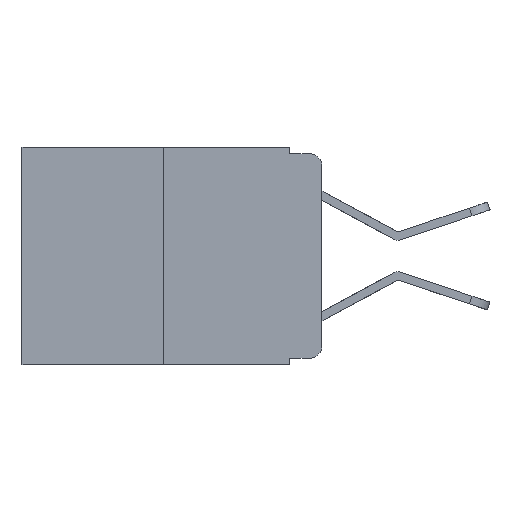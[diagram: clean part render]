
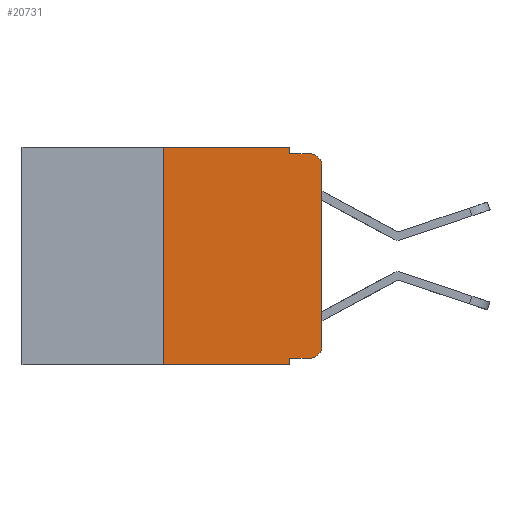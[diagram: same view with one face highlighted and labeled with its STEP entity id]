
A CAD part, left-side view. The second image highlights one B-rep face of the part: STEP entity #20731.
In plain terms, the highlighted planar face has unit normal (-1, 0, 0).
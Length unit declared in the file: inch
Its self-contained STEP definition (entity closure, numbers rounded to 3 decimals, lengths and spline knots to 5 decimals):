
#148 = VERTEX_POINT ( 'NONE', #4072 ) ;
#224 = DIRECTION ( 'NONE',  ( 0., 0., -1. ) ) ;
#341 = DIRECTION ( 'NONE',  ( 0., 0., -1. ) ) ;
#916 = VECTOR ( 'NONE', #18086, 39.37008 ) ;
#939 = EDGE_LOOP ( 'NONE', ( #4129, #20770, #5629, #3543, #6259, #16792, #4773, #17685, #23630, #23408 ) ) ;
#2148 = VERTEX_POINT ( 'NONE', #23301 ) ;
#2504 = LINE ( 'NONE', #6174, #8136 ) ;
#2553 = LINE ( 'NONE', #23036, #12594 ) ;
#3017 = CARTESIAN_POINT ( 'NONE',  ( 0., 0.473, 0. ) ) ;
#3543 = ORIENTED_EDGE ( 'NONE', *, *, #16401, .F. ) ;
#4072 = CARTESIAN_POINT ( 'NONE',  ( 0., 0.051, -0.01 ) ) ;
#4129 = ORIENTED_EDGE ( 'NONE', *, *, #15469, .T. ) ;
#4682 = VERTEX_POINT ( 'NONE', #21403 ) ;
#4773 = ORIENTED_EDGE ( 'NONE', *, *, #18448, .T. ) ;
#4928 = VERTEX_POINT ( 'NONE', #19489 ) ;
#4990 = AXIS2_PLACEMENT_3D ( 'NONE', #18432, #7250, #20255 ) ;
#5586 = VERTEX_POINT ( 'NONE', #23264 ) ;
#5629 = ORIENTED_EDGE ( 'NONE', *, *, #20079, .F. ) ;
#6174 = CARTESIAN_POINT ( 'NONE',  ( 0., 0.473, 0. ) ) ;
#6259 = ORIENTED_EDGE ( 'NONE', *, *, #19309, .F. ) ;
#6754 = VERTEX_POINT ( 'NONE', #23220 ) ;
#7192 = CIRCLE ( 'NONE', #4990, 0.02 ) ;
#7250 = DIRECTION ( 'NONE',  ( -1., 0., 0. ) ) ;
#8136 = VECTOR ( 'NONE', #15414, 39.37008 ) ;
#8357 = CARTESIAN_POINT ( 'NONE',  ( 0., 0.25, -0.343 ) ) ;
#8527 = EDGE_CURVE ( 'NONE', #14965, #6754, #18159, .T. ) ;
#8721 = DIRECTION ( 'NONE',  ( 0., 0., -1. ) ) ;
#9644 = CARTESIAN_POINT ( 'NONE',  ( 0., 0.051, 0. ) ) ;
#10605 = EDGE_CURVE ( 'NONE', #5586, #11191, #13725, .T. ) ;
#10972 = LINE ( 'NONE', #21681, #916 ) ;
#11020 = VECTOR ( 'NONE', #224, 39.37008 ) ;
#11191 = VERTEX_POINT ( 'NONE', #15287 ) ;
#11338 = CARTESIAN_POINT ( 'NONE',  ( 0., 0.02, -0.333 ) ) ;
#11652 = VECTOR ( 'NONE', #16606, 39.37008 ) ;
#11673 = DIRECTION ( 'NONE',  ( -1., 0., 0. ) ) ;
#12017 = DIRECTION ( 'NONE',  ( 0., -1., 0. ) ) ;
#12422 = PLANE ( 'NONE',  #21670 ) ;
#12594 = VECTOR ( 'NONE', #12017, 39.37008 ) ;
#13725 = LINE ( 'NONE', #19593, #22347 ) ;
#14134 = VECTOR ( 'NONE', #20809, 39.37008 ) ;
#14173 = CARTESIAN_POINT ( 'NONE',  ( 0., 0., -0.03 ) ) ;
#14273 = VECTOR ( 'NONE', #17667, 39.37008 ) ;
#14535 = FACE_OUTER_BOUND ( 'NONE', #939, .T. ) ;
#14965 = VERTEX_POINT ( 'NONE', #11338 ) ;
#15287 = CARTESIAN_POINT ( 'NONE',  ( 0., 0.051, -0.343 ) ) ;
#15414 = DIRECTION ( 'NONE',  ( 0., -1., 0. ) ) ;
#15469 = EDGE_CURVE ( 'NONE', #6754, #20162, #16607, .T. ) ;
#15896 = LINE ( 'NONE', #18980, #14134 ) ;
#16401 = EDGE_CURVE ( 'NONE', #4682, #148, #16561, .T. ) ;
#16561 = LINE ( 'NONE', #9644, #11020 ) ;
#16606 = DIRECTION ( 'NONE',  ( 0., 0., 1. ) ) ;
#16607 = LINE ( 'NONE', #20129, #11652 ) ;
#16792 = ORIENTED_EDGE ( 'NONE', *, *, #22965, .F. ) ;
#17326 = EDGE_CURVE ( 'NONE', #5586, #14965, #10972, .T. ) ;
#17667 = DIRECTION ( 'NONE',  ( 0., -1., 0. ) ) ;
#17685 = ORIENTED_EDGE ( 'NONE', *, *, #10605, .F. ) ;
#17842 = DIRECTION ( 'NONE',  ( 0., 0., -1. ) ) ;
#18086 = DIRECTION ( 'NONE',  ( 0., -1., 0. ) ) ;
#18159 = CIRCLE ( 'NONE', #22554, 0.02 ) ;
#18432 = CARTESIAN_POINT ( 'NONE',  ( 0., 0.02, -0.03 ) ) ;
#18448 = EDGE_CURVE ( 'NONE', #21267, #11191, #2553, .T. ) ;
#18980 = CARTESIAN_POINT ( 'NONE',  ( 0., 0.25, 0. ) ) ;
#19172 = LINE ( 'NONE', #23061, #14273 ) ;
#19309 = EDGE_CURVE ( 'NONE', #4928, #4682, #2504, .T. ) ;
#19489 = CARTESIAN_POINT ( 'NONE',  ( 0., 0.25, 0. ) ) ;
#19593 = CARTESIAN_POINT ( 'NONE',  ( 0., 0.051, 0. ) ) ;
#19864 = DIRECTION ( 'NONE',  ( 1., 0., 0. ) ) ;
#20079 = EDGE_CURVE ( 'NONE', #148, #2148, #19172, .T. ) ;
#20129 = CARTESIAN_POINT ( 'NONE',  ( 0., 0., 0. ) ) ;
#20162 = VERTEX_POINT ( 'NONE', #14173 ) ;
#20255 = DIRECTION ( 'NONE',  ( 0., 0., -1. ) ) ;
#20731 = ADVANCED_FACE ( 'NONE', ( #14535 ), #12422, .F. ) ;
#20770 = ORIENTED_EDGE ( 'NONE', *, *, #20847, .T. ) ;
#20809 = DIRECTION ( 'NONE',  ( 0., 0., 1. ) ) ;
#20847 = EDGE_CURVE ( 'NONE', #20162, #2148, #7192, .T. ) ;
#21267 = VERTEX_POINT ( 'NONE', #8357 ) ;
#21403 = CARTESIAN_POINT ( 'NONE',  ( 0., 0.051, 0. ) ) ;
#21670 = AXIS2_PLACEMENT_3D ( 'NONE', #3017, #19864, #8721 ) ;
#21681 = CARTESIAN_POINT ( 'NONE',  ( 0., 0.051, -0.333 ) ) ;
#22347 = VECTOR ( 'NONE', #17842, 39.37008 ) ;
#22554 = AXIS2_PLACEMENT_3D ( 'NONE', #22699, #11673, #341 ) ;
#22699 = CARTESIAN_POINT ( 'NONE',  ( 0., 0.02, -0.313 ) ) ;
#22965 = EDGE_CURVE ( 'NONE', #21267, #4928, #15896, .T. ) ;
#23036 = CARTESIAN_POINT ( 'NONE',  ( 0., 0.473, -0.343 ) ) ;
#23061 = CARTESIAN_POINT ( 'NONE',  ( 0., 0.051, -0.01 ) ) ;
#23220 = CARTESIAN_POINT ( 'NONE',  ( 0., 0., -0.313 ) ) ;
#23264 = CARTESIAN_POINT ( 'NONE',  ( 0., 0.051, -0.333 ) ) ;
#23301 = CARTESIAN_POINT ( 'NONE',  ( 0., 0.02, -0.01 ) ) ;
#23408 = ORIENTED_EDGE ( 'NONE', *, *, #8527, .T. ) ;
#23630 = ORIENTED_EDGE ( 'NONE', *, *, #17326, .T. ) ;
